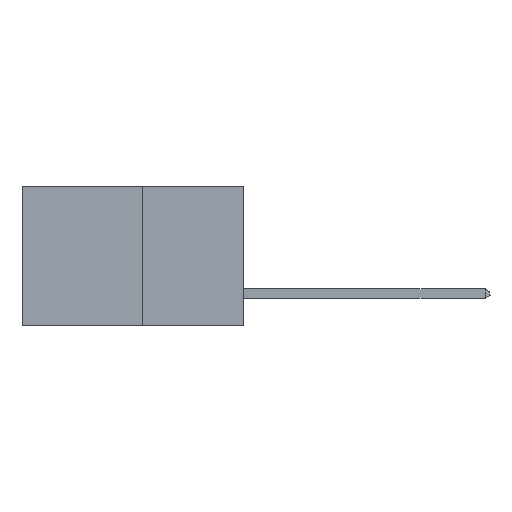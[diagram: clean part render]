
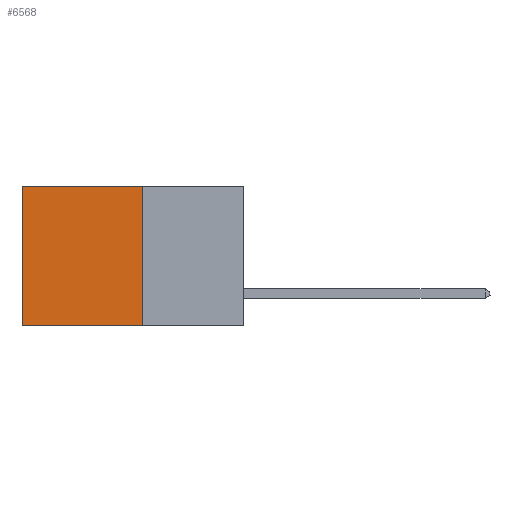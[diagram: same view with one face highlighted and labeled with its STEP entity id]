
A CAD part, left-side view. The second image highlights one B-rep face of the part: STEP entity #6568.
In plain terms, the highlighted planar face has unit normal (-1, 0, 0).
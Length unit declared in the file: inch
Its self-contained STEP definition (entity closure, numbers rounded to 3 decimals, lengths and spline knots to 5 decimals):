
#321 = CARTESIAN_POINT ( 'NONE',  ( 0.277, 0.59, 0. ) ) ;
#455 = ORIENTED_EDGE ( 'NONE', *, *, #5494, .F. ) ;
#694 = DIRECTION ( 'NONE',  ( 0., 0., -1. ) ) ;
#900 = FACE_OUTER_BOUND ( 'NONE', #2107, .T. ) ;
#1516 = CARTESIAN_POINT ( 'NONE',  ( 0.277, 0.27, -0.37 ) ) ;
#1854 = EDGE_CURVE ( 'NONE', #8282, #5527, #8387, .T. ) ;
#2107 = EDGE_LOOP ( 'NONE', ( #2954, #6315, #455, #6550 ) ) ;
#2231 = VERTEX_POINT ( 'NONE', #321 ) ;
#2429 = VERTEX_POINT ( 'NONE', #3019 ) ;
#2818 = VECTOR ( 'NONE', #7919, 39.37008 ) ;
#2954 = ORIENTED_EDGE ( 'NONE', *, *, #7428, .T. ) ;
#3019 = CARTESIAN_POINT ( 'NONE',  ( 0.277, 0.27, 0. ) ) ;
#3464 = CARTESIAN_POINT ( 'NONE',  ( 0.277, 0.27, 0. ) ) ;
#3997 = DIRECTION ( 'NONE',  ( 0., 0., -1. ) ) ;
#4074 = CARTESIAN_POINT ( 'NONE',  ( 0.277, 0.59, -0.37 ) ) ;
#4191 = LINE ( 'NONE', #5544, #6124 ) ;
#4286 = EDGE_CURVE ( 'NONE', #2429, #2231, #8527, .T. ) ;
#4371 = AXIS2_PLACEMENT_3D ( 'NONE', #1516, #8114, #3997 ) ;
#5046 = VECTOR ( 'NONE', #8858, 39.37008 ) ;
#5494 = EDGE_CURVE ( 'NONE', #2429, #8282, #4191, .T. ) ;
#5527 = VERTEX_POINT ( 'NONE', #4074 ) ;
#5544 = CARTESIAN_POINT ( 'NONE',  ( 0.277, 0.27, -0.37 ) ) ;
#6124 = VECTOR ( 'NONE', #694, 39.37008 ) ;
#6205 = VECTOR ( 'NONE', #8776, 39.37008 ) ;
#6315 = ORIENTED_EDGE ( 'NONE', *, *, #1854, .F. ) ;
#6550 = ORIENTED_EDGE ( 'NONE', *, *, #4286, .T. ) ;
#6568 = ADVANCED_FACE ( 'NONE', ( #900 ), #7473, .F. ) ;
#7428 = EDGE_CURVE ( 'NONE', #2231, #5527, #9310, .T. ) ;
#7473 = PLANE ( 'NONE',  #4371 ) ;
#7919 = DIRECTION ( 'NONE',  ( 0., 1., 0. ) ) ;
#8114 = DIRECTION ( 'NONE',  ( 1., 0., 0. ) ) ;
#8181 = CARTESIAN_POINT ( 'NONE',  ( 0.277, 0.59, -0.37 ) ) ;
#8200 = CARTESIAN_POINT ( 'NONE',  ( 0.277, 0.27, -0.37 ) ) ;
#8282 = VERTEX_POINT ( 'NONE', #8200 ) ;
#8387 = LINE ( 'NONE', #8572, #2818 ) ;
#8527 = LINE ( 'NONE', #3464, #5046 ) ;
#8572 = CARTESIAN_POINT ( 'NONE',  ( 0.277, 0.27, -0.37 ) ) ;
#8776 = DIRECTION ( 'NONE',  ( 0., 0., -1. ) ) ;
#8858 = DIRECTION ( 'NONE',  ( 0., 1., 0. ) ) ;
#9310 = LINE ( 'NONE', #8181, #6205 ) ;
